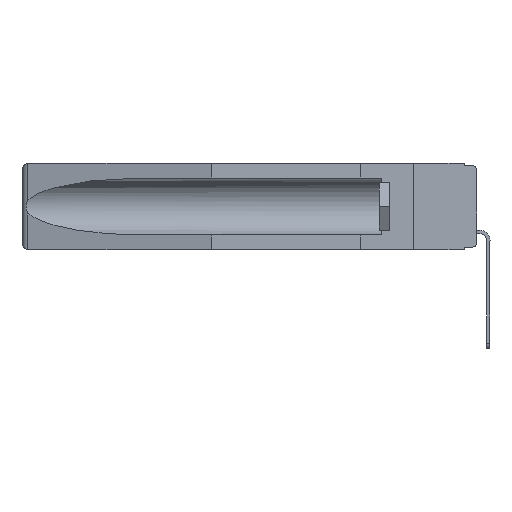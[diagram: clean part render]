
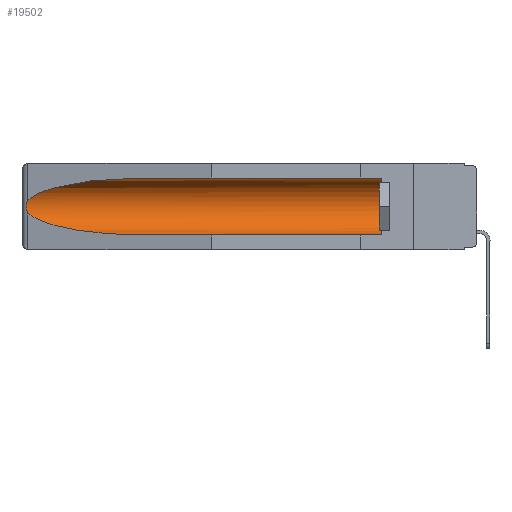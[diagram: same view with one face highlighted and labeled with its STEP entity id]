
A CAD part, left-side view. The second image highlights one B-rep face of the part: STEP entity #19502.
In plain terms, the highlighted cylindrical face has radius 2.857 mm (diameter 5.715 mm), a partial arc.
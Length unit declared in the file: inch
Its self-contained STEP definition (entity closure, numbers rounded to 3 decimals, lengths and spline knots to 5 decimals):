
#866 = DIRECTION ( 'NONE',  ( 0., 0., 1. ) ) ;
#867 =( BOUNDED_CURVE ( )  B_SPLINE_CURVE ( 3, ( #19867, #22048, #10671, #18348 ),
 .UNSPECIFIED., .F., .T. ) 
 B_SPLINE_CURVE_WITH_KNOTS ( ( 4, 4 ),
 ( 4.71239, 6.08839 ),
 .UNSPECIFIED. ) 
 CURVE ( )  GEOMETRIC_REPRESENTATION_ITEM ( )  RATIONAL_B_SPLINE_CURVE ( ( 1., 0.848, 0.848, 1. ) ) 
 REPRESENTATION_ITEM ( '' )  );
#1139 = DIRECTION ( 'NONE',  ( 0., 1., 0. ) ) ;
#1374 = EDGE_CURVE ( 'NONE', #16772, #9976, #2235, .T. ) ;
#1611 =( BOUNDED_CURVE ( )  B_SPLINE_CURVE ( 3, ( #23521, #14227, #8750, #6820 ),
 .UNSPECIFIED., .F., .F. ) 
 B_SPLINE_CURVE_WITH_KNOTS ( ( 4, 4 ),
 ( 0.1948, 1.5708 ),
 .UNSPECIFIED. ) 
 CURVE ( )  GEOMETRIC_REPRESENTATION_ITEM ( )  RATIONAL_B_SPLINE_CURVE ( ( 1., 0.848, 0.848, 1. ) ) 
 REPRESENTATION_ITEM ( '' )  );
#1950 = CARTESIAN_POINT ( 'NONE',  ( 0.155, 1.07973, -0.284 ) ) ;
#2029 = DIRECTION ( 'NONE',  ( 0., 1., 0. ) ) ;
#2235 = LINE ( 'NONE', #15150, #21538 ) ;
#3884 = EDGE_CURVE ( 'NONE', #13692, #9976, #1611, .T. ) ;
#4348 = CARTESIAN_POINT ( 'NONE',  ( 0.2673, 1.53269, -0.17917 ) ) ;
#4427 = CARTESIAN_POINT ( 'NONE',  ( 0.26654, 1.53092, -0.15636 ) ) ;
#5643 = CARTESIAN_POINT ( 'NONE',  ( 0.155, 1.07973, -0.059 ) ) ;
#5919 = LINE ( 'NONE', #10154, #12863 ) ;
#6103 = CARTESIAN_POINT ( 'NONE',  ( 0.2675, 1.53308, -0.16763 ) ) ;
#6152 = VERTEX_POINT ( 'NONE', #5643 ) ;
#6648 = CARTESIAN_POINT ( 'NONE',  ( 0.26537, 1.52718, -0.14972 ) ) ;
#6820 = CARTESIAN_POINT ( 'NONE',  ( 0.155, 1.07973, -0.284 ) ) ;
#7833 = EDGE_CURVE ( 'NONE', #6152, #8600, #867, .T. ) ;
#7844 = AXIS2_PLACEMENT_3D ( 'NONE', #20590, #9536, #8019 ) ;
#8019 = DIRECTION ( 'NONE',  ( 0., 0., 1. ) ) ;
#8212 = CARTESIAN_POINT ( 'NONE',  ( 0.26537, 1.52718, -0.14972 ) ) ;
#8600 = VERTEX_POINT ( 'NONE', #6648 ) ;
#8750 = CARTESIAN_POINT ( 'NONE',  ( 0.21114, 1.30732, -0.284 ) ) ;
#9536 = DIRECTION ( 'NONE',  ( 0., -1., 0. ) ) ;
#9964 = CARTESIAN_POINT ( 'NONE',  ( 0.155, -0.30754, -0.1715 ) ) ;
#9976 = VERTEX_POINT ( 'NONE', #1950 ) ;
#10062 = CARTESIAN_POINT ( 'NONE',  ( 0.155, 0.126, -0.059 ) ) ;
#10154 = CARTESIAN_POINT ( 'NONE',  ( 0.155, -0.30754, -0.059 ) ) ;
#10671 = CARTESIAN_POINT ( 'NONE',  ( 0.25451, 1.48313, -0.09465 ) ) ;
#10904 = EDGE_LOOP ( 'NONE', ( #14047, #22465, #19806, #11446, #18758, #22180 ) ) ;
#11446 = ORIENTED_EDGE ( 'NONE', *, *, #1374, .F. ) ;
#11826 = CARTESIAN_POINT ( 'NONE',  ( 0.26537, 1.52718, -0.19328 ) ) ;
#11907 = CARTESIAN_POINT ( 'NONE',  ( 0.26655, 1.53094, -0.18657 ) ) ;
#12863 = VECTOR ( 'NONE', #1139, 39.37008 ) ;
#13692 = VERTEX_POINT ( 'NONE', #22340 ) ;
#14047 = ORIENTED_EDGE ( 'NONE', *, *, #7833, .T. ) ;
#14219 = CIRCLE ( 'NONE', #7844, 0.1125 ) ;
#14227 = CARTESIAN_POINT ( 'NONE',  ( 0.25451, 1.48313, -0.24835 ) ) ;
#14750 = B_SPLINE_CURVE_WITH_KNOTS ( 'NONE', 3,
 ( #8212, #21014, #4427, #17335, #6103, #15545, #4348, #11907, #22879, #11826 ),
 .UNSPECIFIED., .F., .F.,
 ( 4, 2, 2, 2, 4 ),
 ( 0., 0.00029, 0.00058, 0.00087, 0.00117 ),
 .UNSPECIFIED. ) ;
#15150 = CARTESIAN_POINT ( 'NONE',  ( 0.155, -0.30754, -0.284 ) ) ;
#15545 = CARTESIAN_POINT ( 'NONE',  ( 0.2675, 1.53308, -0.17534 ) ) ;
#15741 = VERTEX_POINT ( 'NONE', #10062 ) ;
#16195 = EDGE_CURVE ( 'NONE', #15741, #6152, #5919, .T. ) ;
#16711 = EDGE_CURVE ( 'NONE', #8600, #13692, #14750, .T. ) ;
#16772 = VERTEX_POINT ( 'NONE', #17410 ) ;
#17315 = EDGE_CURVE ( 'NONE', #16772, #15741, #14219, .T. ) ;
#17335 = CARTESIAN_POINT ( 'NONE',  ( 0.2673, 1.5327, -0.16383 ) ) ;
#17410 = CARTESIAN_POINT ( 'NONE',  ( 0.155, 0.126, -0.284 ) ) ;
#18348 = CARTESIAN_POINT ( 'NONE',  ( 0.26537, 1.52718, -0.14972 ) ) ;
#18758 = ORIENTED_EDGE ( 'NONE', *, *, #17315, .T. ) ;
#19502 = ADVANCED_FACE ( 'NONE', ( #20398 ), #20095, .F. ) ;
#19806 = ORIENTED_EDGE ( 'NONE', *, *, #3884, .T. ) ;
#19867 = CARTESIAN_POINT ( 'NONE',  ( 0.155, 1.07973, -0.059 ) ) ;
#20095 = CYLINDRICAL_SURFACE ( 'NONE', #20998, 0.1125 ) ;
#20398 = FACE_OUTER_BOUND ( 'NONE', #10904, .T. ) ;
#20590 = CARTESIAN_POINT ( 'NONE',  ( 0.155, 0.126, -0.1715 ) ) ;
#20998 = AXIS2_PLACEMENT_3D ( 'NONE', #9964, #22795, #866 ) ;
#21014 = CARTESIAN_POINT ( 'NONE',  ( 0.26597, 1.52961, -0.15275 ) ) ;
#21538 = VECTOR ( 'NONE', #2029, 39.37008 ) ;
#22048 = CARTESIAN_POINT ( 'NONE',  ( 0.21114, 1.30732, -0.059 ) ) ;
#22180 = ORIENTED_EDGE ( 'NONE', *, *, #16195, .T. ) ;
#22340 = CARTESIAN_POINT ( 'NONE',  ( 0.26537, 1.52718, -0.19328 ) ) ;
#22465 = ORIENTED_EDGE ( 'NONE', *, *, #16711, .T. ) ;
#22795 = DIRECTION ( 'NONE',  ( 0., 1., 0. ) ) ;
#22879 = CARTESIAN_POINT ( 'NONE',  ( 0.26597, 1.5296, -0.19026 ) ) ;
#23521 = CARTESIAN_POINT ( 'NONE',  ( 0.26537, 1.52718, -0.19328 ) ) ;
